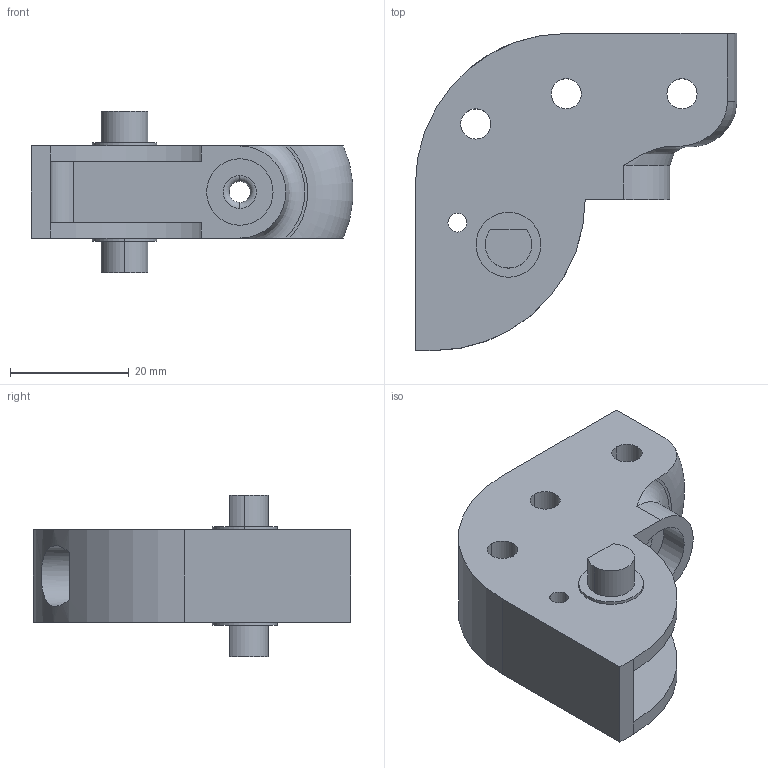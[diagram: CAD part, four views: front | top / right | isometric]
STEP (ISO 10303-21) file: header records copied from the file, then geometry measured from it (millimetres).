
FILE_DESCRIPTION (( 'STEP AP214' ), '1' );
FILE_NAME ('hammer_body.STEP', '2013-06-07T17:15:42', ( 'Asher' ), ( '' ), 'SwSTEP 2.0', 'SolidWorks 2013', '' );
FILE_SCHEMA (( 'AUTOMOTIVE_DESIGN' ));
Length unit declared in the file: millimetre
Products named in the file (1): hammer_body
Bounding box: 54.06 x 53.34 x 27.18 mm (x, y, z)
Volume: 21727 mm3; surface area: 8978.4 mm2
Topology: 1 solids, 1 shells, 54 faces, 134 edges, 88 vertices
Faces by surface type: cylinder 32, plane 18, torus 4
Entity records: 1797 total; most frequent: CARTESIAN_POINT 397, DIRECTION 304, ORIENTED_EDGE 268, EDGE_CURVE 134, AXIS2_PLACEMENT_3D 122, VERTEX_POINT 88, EDGE_LOOP 72, CIRCLE 67
